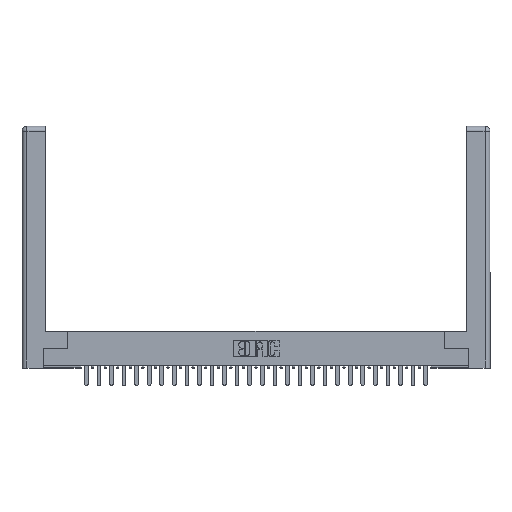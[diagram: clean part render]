
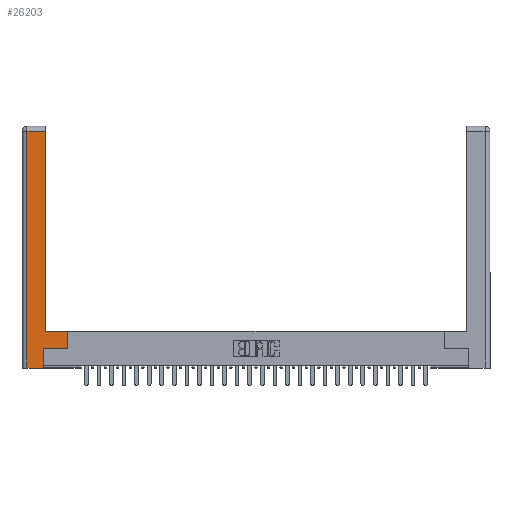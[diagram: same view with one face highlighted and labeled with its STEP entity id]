
A CAD part, top view. The second image highlights one B-rep face of the part: STEP entity #26203.
In plain terms, the highlighted planar face has unit normal (0, 0, 1).
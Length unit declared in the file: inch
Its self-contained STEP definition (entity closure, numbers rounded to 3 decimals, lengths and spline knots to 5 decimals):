
#335 = LINE ( 'NONE', #27639, #12009 ) ;
#531 = AXIS2_PLACEMENT_3D ( 'NONE', #28606, #28490, #1798 ) ;
#1247 = CARTESIAN_POINT ( 'NONE',  ( 0.265, 0., 0. ) ) ;
#1523 = VECTOR ( 'NONE', #15257, 39.37008 ) ;
#1688 = VERTEX_POINT ( 'NONE', #4405 ) ;
#1798 = DIRECTION ( 'NONE',  ( -1., 0., 0. ) ) ;
#2196 = EDGE_CURVE ( 'NONE', #14786, #28889, #26257, .T. ) ;
#2206 = VECTOR ( 'NONE', #6368, 39.37008 ) ;
#3770 = CARTESIAN_POINT ( 'NONE',  ( 0.565, 0.245, 0. ) ) ;
#3895 = VERTEX_POINT ( 'NONE', #9168 ) ;
#4405 = CARTESIAN_POINT ( 'NONE',  ( 0.0615, 2.94, 0. ) ) ;
#6307 = ORIENTED_EDGE ( 'NONE', *, *, #11079, .T. ) ;
#6368 = DIRECTION ( 'NONE',  ( 1., 0., 0. ) ) ;
#6824 = EDGE_CURVE ( 'NONE', #23587, #33392, #26791, .T. ) ;
#7169 = CARTESIAN_POINT ( 'NONE',  ( 0.0615, 2.94, 0. ) ) ;
#7221 = DIRECTION ( 'NONE',  ( 0., 1., 0. ) ) ;
#7773 = ORIENTED_EDGE ( 'NONE', *, *, #9708, .T. ) ;
#7933 = CARTESIAN_POINT ( 'NONE',  ( 0.265, 0.245, 0. ) ) ;
#8045 = CARTESIAN_POINT ( 'NONE',  ( 0.295, 0.45, 0. ) ) ;
#8406 = VECTOR ( 'NONE', #7221, 39.37008 ) ;
#8626 = DIRECTION ( 'NONE',  ( 0., 1., 0. ) ) ;
#9168 = CARTESIAN_POINT ( 'NONE',  ( 0.0615, 0., 0. ) ) ;
#9708 = EDGE_CURVE ( 'NONE', #33392, #1688, #23322, .T. ) ;
#10403 = CARTESIAN_POINT ( 'NONE',  ( 0.0615, 0., 0. ) ) ;
#10741 = DIRECTION ( 'NONE',  ( 0., -1., 0. ) ) ;
#11079 = EDGE_CURVE ( 'NONE', #11573, #30187, #335, .T. ) ;
#11573 = VERTEX_POINT ( 'NONE', #22449 ) ;
#12009 = VECTOR ( 'NONE', #8626, 39.37008 ) ;
#13185 = ORIENTED_EDGE ( 'NONE', *, *, #24789, .T. ) ;
#13289 = VECTOR ( 'NONE', #15114, 39.37008 ) ;
#14724 = CARTESIAN_POINT ( 'NONE',  ( 0.295, 0.45, 0. ) ) ;
#14786 = VERTEX_POINT ( 'NONE', #24205 ) ;
#15114 = DIRECTION ( 'NONE',  ( -1., 0., 0. ) ) ;
#15257 = DIRECTION ( 'NONE',  ( 1., 0., 0. ) ) ;
#15488 = CARTESIAN_POINT ( 'NONE',  ( 0.565, 0.45, 0. ) ) ;
#16553 = LINE ( 'NONE', #1247, #1523 ) ;
#18439 = LINE ( 'NONE', #3770, #2206 ) ;
#19104 = EDGE_CURVE ( 'NONE', #3895, #11573, #16553, .T. ) ;
#20862 = VECTOR ( 'NONE', #24991, 39.37008 ) ;
#21951 = LINE ( 'NONE', #10403, #28196 ) ;
#22020 = CARTESIAN_POINT ( 'NONE',  ( 0.565, 0.45, 0. ) ) ;
#22449 = CARTESIAN_POINT ( 'NONE',  ( 0.265, 0., 0. ) ) ;
#22666 = DIRECTION ( 'NONE',  ( -1., 0., 0. ) ) ;
#23322 = LINE ( 'NONE', #7169, #13289 ) ;
#23380 = PLANE ( 'NONE',  #531 ) ;
#23587 = VERTEX_POINT ( 'NONE', #8045 ) ;
#24037 = EDGE_CURVE ( 'NONE', #28889, #23587, #32350, .T. ) ;
#24205 = CARTESIAN_POINT ( 'NONE',  ( 0.565, 0.245, 0. ) ) ;
#24789 = EDGE_CURVE ( 'NONE', #1688, #3895, #21951, .T. ) ;
#24991 = DIRECTION ( 'NONE',  ( 0., 1., 0. ) ) ;
#25764 = CARTESIAN_POINT ( 'NONE',  ( 0.295, 3., 0. ) ) ;
#26203 = ADVANCED_FACE ( 'NONE', ( #26858 ), #23380, .F. ) ;
#26257 = LINE ( 'NONE', #22020, #20862 ) ;
#26427 = EDGE_LOOP ( 'NONE', ( #33052, #7773, #13185, #30739, #6307, #28642, #33225, #29418 ) ) ;
#26791 = LINE ( 'NONE', #25764, #8406 ) ;
#26858 = FACE_OUTER_BOUND ( 'NONE', #26427, .T. ) ;
#27639 = CARTESIAN_POINT ( 'NONE',  ( 0.265, 0.245, 0. ) ) ;
#27736 = CARTESIAN_POINT ( 'NONE',  ( 0.295, 2.94, 0. ) ) ;
#28196 = VECTOR ( 'NONE', #10741, 39.37008 ) ;
#28490 = DIRECTION ( 'NONE',  ( 0., 0., -1. ) ) ;
#28606 = CARTESIAN_POINT ( 'NONE',  ( 0., 0., 0. ) ) ;
#28642 = ORIENTED_EDGE ( 'NONE', *, *, #32322, .T. ) ;
#28889 = VERTEX_POINT ( 'NONE', #15488 ) ;
#29418 = ORIENTED_EDGE ( 'NONE', *, *, #24037, .T. ) ;
#30187 = VERTEX_POINT ( 'NONE', #7933 ) ;
#30696 = VECTOR ( 'NONE', #22666, 39.37008 ) ;
#30739 = ORIENTED_EDGE ( 'NONE', *, *, #19104, .T. ) ;
#32322 = EDGE_CURVE ( 'NONE', #30187, #14786, #18439, .T. ) ;
#32350 = LINE ( 'NONE', #14724, #30696 ) ;
#33052 = ORIENTED_EDGE ( 'NONE', *, *, #6824, .T. ) ;
#33225 = ORIENTED_EDGE ( 'NONE', *, *, #2196, .T. ) ;
#33392 = VERTEX_POINT ( 'NONE', #27736 ) ;
